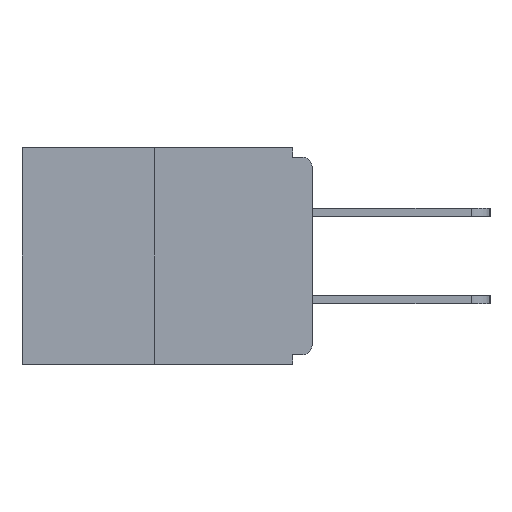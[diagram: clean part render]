
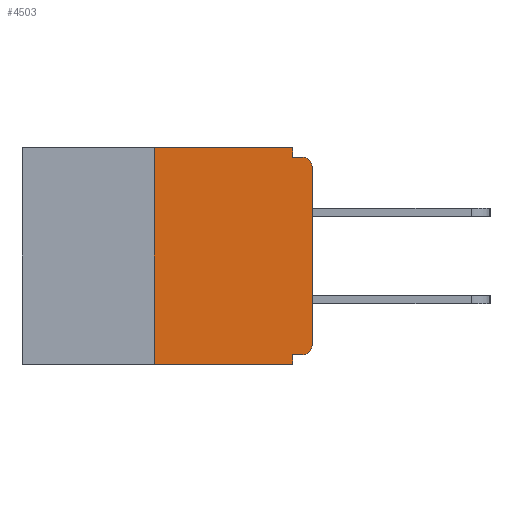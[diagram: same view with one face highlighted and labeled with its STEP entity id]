
A CAD part, left-side view. The second image highlights one B-rep face of the part: STEP entity #4503.
In plain terms, the highlighted planar face has unit normal (-1, 0, 0).
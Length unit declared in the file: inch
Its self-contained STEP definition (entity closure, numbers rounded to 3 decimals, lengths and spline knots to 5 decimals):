
#398 = VERTEX_POINT ( 'NONE', #7686 ) ;
#959 = DIRECTION ( 'NONE',  ( 0., 0., -1. ) ) ;
#1013 = ORIENTED_EDGE ( 'NONE', *, *, #1456, .F. ) ;
#1135 = VECTOR ( 'NONE', #19571, 39.37008 ) ;
#1456 = EDGE_CURVE ( 'NONE', #23361, #21478, #27269, .T. ) ;
#2896 = ORIENTED_EDGE ( 'NONE', *, *, #14859, .F. ) ;
#3021 = DIRECTION ( 'NONE',  ( 0., 0., 1. ) ) ;
#3662 = CARTESIAN_POINT ( 'NONE',  ( 0., 0.031, 0. ) ) ;
#3748 = LINE ( 'NONE', #12268, #20678 ) ;
#3879 = DIRECTION ( 'NONE',  ( 0., -1., 0. ) ) ;
#4262 = FACE_OUTER_BOUND ( 'NONE', #25799, .T. ) ;
#4377 = CARTESIAN_POINT ( 'NONE',  ( 0., 0.031, -0.328 ) ) ;
#4503 = ADVANCED_FACE ( 'NONE', ( #4262 ), #8892, .F. ) ;
#4612 = EDGE_CURVE ( 'NONE', #17622, #8807, #15879, .T. ) ;
#4653 = DIRECTION ( 'NONE',  ( 0., 0., -1. ) ) ;
#4816 = DIRECTION ( 'NONE',  ( 1., 0., 0. ) ) ;
#4949 = CARTESIAN_POINT ( 'NONE',  ( 0., 0., 0. ) ) ;
#4956 = CIRCLE ( 'NONE', #22391, 0.015 ) ;
#5172 = LINE ( 'NONE', #13710, #21394 ) ;
#6415 = ORIENTED_EDGE ( 'NONE', *, *, #10672, .F. ) ;
#6761 = EDGE_CURVE ( 'NONE', #14908, #17622, #9662, .T. ) ;
#7686 = CARTESIAN_POINT ( 'NONE',  ( 0., 0.25, -0.343 ) ) ;
#8101 = VERTEX_POINT ( 'NONE', #15381 ) ;
#8140 = ORIENTED_EDGE ( 'NONE', *, *, #18659, .F. ) ;
#8577 = ORIENTED_EDGE ( 'NONE', *, *, #26415, .T. ) ;
#8713 = LINE ( 'NONE', #19070, #15318 ) ;
#8807 = VERTEX_POINT ( 'NONE', #15004 ) ;
#8892 = PLANE ( 'NONE',  #22102 ) ;
#9662 = CIRCLE ( 'NONE', #17277, 0.015 ) ;
#9902 = DIRECTION ( 'NONE',  ( 0., -1., 0. ) ) ;
#10446 = ORIENTED_EDGE ( 'NONE', *, *, #12694, .T. ) ;
#10672 = EDGE_CURVE ( 'NONE', #14908, #26336, #5172, .T. ) ;
#11047 = VECTOR ( 'NONE', #21152, 39.37008 ) ;
#12025 = CARTESIAN_POINT ( 'NONE',  ( 0., 0.031, -0.015 ) ) ;
#12268 = CARTESIAN_POINT ( 'NONE',  ( 0., 0.46, -0.343 ) ) ;
#12694 = EDGE_CURVE ( 'NONE', #398, #8101, #3748, .T. ) ;
#12896 = DIRECTION ( 'NONE',  ( 0., 0., 1. ) ) ;
#13622 = DIRECTION ( 'NONE',  ( -1., 0., 0. ) ) ;
#13669 = LINE ( 'NONE', #18034, #16758 ) ;
#13710 = CARTESIAN_POINT ( 'NONE',  ( 0., 0., -0.328 ) ) ;
#14626 = ORIENTED_EDGE ( 'NONE', *, *, #20782, .F. ) ;
#14694 = ORIENTED_EDGE ( 'NONE', *, *, #20872, .F. ) ;
#14859 = EDGE_CURVE ( 'NONE', #17276, #23361, #27477, .T. ) ;
#14908 = VERTEX_POINT ( 'NONE', #23946 ) ;
#15004 = CARTESIAN_POINT ( 'NONE',  ( 0., 0., -0.03 ) ) ;
#15095 = CARTESIAN_POINT ( 'NONE',  ( 0., 0.46, 0. ) ) ;
#15165 = DIRECTION ( 'NONE',  ( -1., 0., 0. ) ) ;
#15318 = VECTOR ( 'NONE', #12896, 39.37008 ) ;
#15381 = CARTESIAN_POINT ( 'NONE',  ( 0., 0.031, -0.343 ) ) ;
#15879 = LINE ( 'NONE', #4949, #17662 ) ;
#16573 = ORIENTED_EDGE ( 'NONE', *, *, #6761, .T. ) ;
#16758 = VECTOR ( 'NONE', #959, 39.37008 ) ;
#17276 = VERTEX_POINT ( 'NONE', #3662 ) ;
#17277 = AXIS2_PLACEMENT_3D ( 'NONE', #24562, #13622, #22017 ) ;
#17294 = CARTESIAN_POINT ( 'NONE',  ( 0., 0.46, 0. ) ) ;
#17564 = DIRECTION ( 'NONE',  ( 0., 0., -1. ) ) ;
#17622 = VERTEX_POINT ( 'NONE', #18591 ) ;
#17662 = VECTOR ( 'NONE', #3021, 39.37008 ) ;
#17686 = CARTESIAN_POINT ( 'NONE',  ( 0., 0.015, -0.03 ) ) ;
#18034 = CARTESIAN_POINT ( 'NONE',  ( 0., 0.031, -0.343 ) ) ;
#18591 = CARTESIAN_POINT ( 'NONE',  ( 0., 0., -0.313 ) ) ;
#18640 = VECTOR ( 'NONE', #3879, 39.37008 ) ;
#18659 = EDGE_CURVE ( 'NONE', #398, #26973, #8713, .T. ) ;
#19070 = CARTESIAN_POINT ( 'NONE',  ( 0., 0.25, 0. ) ) ;
#19571 = DIRECTION ( 'NONE',  ( 0., -1., 0. ) ) ;
#20161 = DIRECTION ( 'NONE',  ( 0., 1., 0. ) ) ;
#20678 = VECTOR ( 'NONE', #9902, 39.37008 ) ;
#20782 = EDGE_CURVE ( 'NONE', #26973, #17276, #22067, .T. ) ;
#20872 = EDGE_CURVE ( 'NONE', #26336, #8101, #13669, .T. ) ;
#20955 = CARTESIAN_POINT ( 'NONE',  ( 0., 0., -0.015 ) ) ;
#21152 = DIRECTION ( 'NONE',  ( 0., 0., -1. ) ) ;
#21394 = VECTOR ( 'NONE', #20161, 39.37008 ) ;
#21478 = VERTEX_POINT ( 'NONE', #25383 ) ;
#22017 = DIRECTION ( 'NONE',  ( 0., 0., -1. ) ) ;
#22067 = LINE ( 'NONE', #15095, #1135 ) ;
#22102 = AXIS2_PLACEMENT_3D ( 'NONE', #17294, #4816, #17564 ) ;
#22391 = AXIS2_PLACEMENT_3D ( 'NONE', #17686, #15165, #4653 ) ;
#23361 = VERTEX_POINT ( 'NONE', #12025 ) ;
#23946 = CARTESIAN_POINT ( 'NONE',  ( 0., 0.015, -0.328 ) ) ;
#24023 = ORIENTED_EDGE ( 'NONE', *, *, #4612, .T. ) ;
#24208 = CARTESIAN_POINT ( 'NONE',  ( 0., 0.25, 0. ) ) ;
#24562 = CARTESIAN_POINT ( 'NONE',  ( 0., 0.015, -0.313 ) ) ;
#25383 = CARTESIAN_POINT ( 'NONE',  ( 0., 0.015, -0.015 ) ) ;
#25635 = CARTESIAN_POINT ( 'NONE',  ( 0., 0.031, 0. ) ) ;
#25799 = EDGE_LOOP ( 'NONE', ( #14626, #8140, #10446, #14694, #6415, #16573, #24023, #8577, #1013, #2896 ) ) ;
#26336 = VERTEX_POINT ( 'NONE', #4377 ) ;
#26415 = EDGE_CURVE ( 'NONE', #8807, #21478, #4956, .T. ) ;
#26973 = VERTEX_POINT ( 'NONE', #24208 ) ;
#27269 = LINE ( 'NONE', #20955, #18640 ) ;
#27477 = LINE ( 'NONE', #25635, #11047 ) ;
